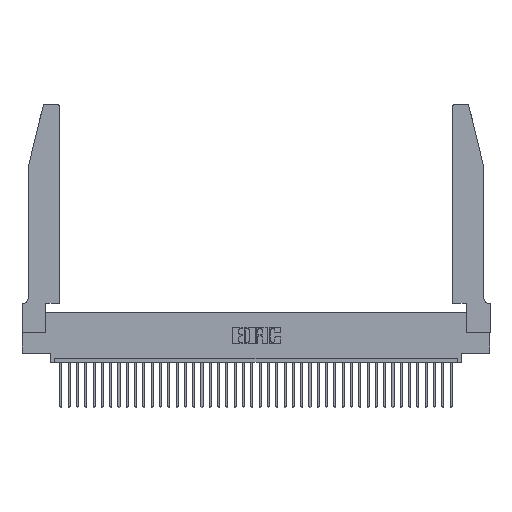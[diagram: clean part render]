
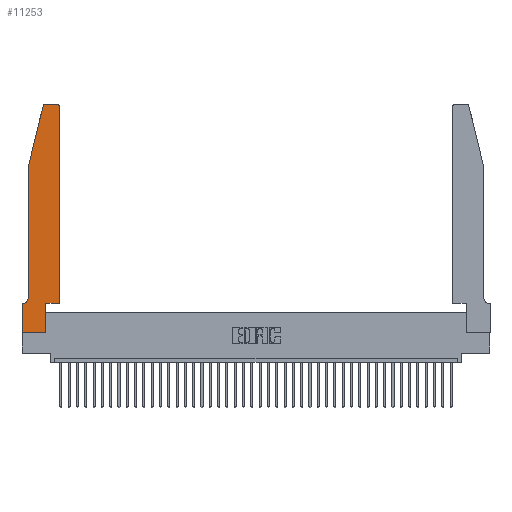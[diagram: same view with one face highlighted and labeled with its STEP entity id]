
A CAD part, top view. The second image highlights one B-rep face of the part: STEP entity #11253.
In plain terms, the highlighted planar face has unit normal (0, 0, 1).
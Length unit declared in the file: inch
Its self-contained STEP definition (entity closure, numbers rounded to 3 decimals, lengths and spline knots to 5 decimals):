
#1245 = EDGE_CURVE ( 'NONE', #4310, #39104, #9713, .T. ) ;
#1651 = CARTESIAN_POINT ( 'NONE',  ( 0.4505, 0.35, 0.37 ) ) ;
#2006 = VECTOR ( 'NONE', #34312, 39.37008 ) ;
#2778 = CARTESIAN_POINT ( 'NONE',  ( 0.2865, 0.35, 0.37 ) ) ;
#3630 = VERTEX_POINT ( 'NONE', #25578 ) ;
#3681 = CARTESIAN_POINT ( 'NONE',  ( 0.0755, 0.35, 0.37 ) ) ;
#4012 = DIRECTION ( 'NONE',  ( 0., 0., 1. ) ) ;
#4310 = VERTEX_POINT ( 'NONE', #18107 ) ;
#4346 = ORIENTED_EDGE ( 'NONE', *, *, #28639, .T. ) ;
#5297 = ORIENTED_EDGE ( 'NONE', *, *, #17449, .T. ) ;
#5808 = VECTOR ( 'NONE', #20023, 39.37008 ) ;
#6354 = ORIENTED_EDGE ( 'NONE', *, *, #28395, .T. ) ;
#6500 = VECTOR ( 'NONE', #26506, 39.37008 ) ;
#6659 = VERTEX_POINT ( 'NONE', #11043 ) ;
#6855 = CARTESIAN_POINT ( 'NONE',  ( 0.0055, 0.42, 0.37 ) ) ;
#7603 = DIRECTION ( 'NONE',  ( 1., 0., 0. ) ) ;
#8012 = CARTESIAN_POINT ( 'NONE',  ( 0.2865, 0.35, 0.37 ) ) ;
#9073 = LINE ( 'NONE', #1651, #40133 ) ;
#9585 = CARTESIAN_POINT ( 'NONE',  ( 0.4505, 2.72, 0.37 ) ) ;
#9713 = LINE ( 'NONE', #3681, #17056 ) ;
#10082 = DIRECTION ( 'NONE',  ( -1., 0., 0. ) ) ;
#10747 = CARTESIAN_POINT ( 'NONE',  ( 0.0755, 2., 0.37 ) ) ;
#11043 = CARTESIAN_POINT ( 'NONE',  ( 0.0755, 0.42, 0.37 ) ) ;
#11166 = CARTESIAN_POINT ( 'NONE',  ( 0.4205, 2.72, 0.37 ) ) ;
#11253 = ADVANCED_FACE ( 'NONE', ( #39019 ), #39192, .T. ) ;
#11574 = CARTESIAN_POINT ( 'NONE',  ( 0.25487, 2.72718, 0.37 ) ) ;
#12387 = LINE ( 'NONE', #8012, #6500 ) ;
#12405 = LINE ( 'NONE', #31126, #32309 ) ;
#12413 = DIRECTION ( 'NONE',  ( 0., -1., 0. ) ) ;
#12526 = DIRECTION ( 'NONE',  ( 0., -1., 0. ) ) ;
#12541 = ORIENTED_EDGE ( 'NONE', *, *, #20061, .T. ) ;
#12631 = CARTESIAN_POINT ( 'NONE',  ( 0., 0., 0.37 ) ) ;
#13280 = DIRECTION ( 'NONE',  ( -1., 0., 0. ) ) ;
#15090 = CIRCLE ( 'NONE', #30594, 0.03 ) ;
#15318 = AXIS2_PLACEMENT_3D ( 'NONE', #11166, #16724, #19846 ) ;
#15451 = ORIENTED_EDGE ( 'NONE', *, *, #33954, .T. ) ;
#16715 = ORIENTED_EDGE ( 'NONE', *, *, #1245, .T. ) ;
#16724 = DIRECTION ( 'NONE',  ( 0., 0., 1. ) ) ;
#17056 = VECTOR ( 'NONE', #10082, 39.37008 ) ;
#17449 = EDGE_CURVE ( 'NONE', #39104, #19648, #27063, .T. ) ;
#17570 = LINE ( 'NONE', #12631, #2006 ) ;
#18107 = CARTESIAN_POINT ( 'NONE',  ( 0.0055, 0.35, 0.37 ) ) ;
#18653 = ORIENTED_EDGE ( 'NONE', *, *, #20448, .T. ) ;
#18967 = ORIENTED_EDGE ( 'NONE', *, *, #39548, .T. ) ;
#19499 = CARTESIAN_POINT ( 'NONE',  ( 0.284, 2.72, 0.37 ) ) ;
#19648 = VERTEX_POINT ( 'NONE', #33228 ) ;
#19846 = DIRECTION ( 'NONE',  ( 1., 0., 0. ) ) ;
#20023 = DIRECTION ( 'NONE',  ( -0.239, -0.971, 0. ) ) ;
#20061 = EDGE_CURVE ( 'NONE', #19648, #30337, #17570, .T. ) ;
#20264 = CARTESIAN_POINT ( 'NONE',  ( 0., 0.35, 0.37 ) ) ;
#20448 = EDGE_CURVE ( 'NONE', #33171, #39243, #30648, .T. ) ;
#20653 = DIRECTION ( 'NONE',  ( 1., 0., 0. ) ) ;
#21458 = LINE ( 'NONE', #29177, #23873 ) ;
#21601 = CARTESIAN_POINT ( 'NONE',  ( 0.284, 2.75, 0.37 ) ) ;
#22159 = AXIS2_PLACEMENT_3D ( 'NONE', #6855, #28776, #13280 ) ;
#22890 = DIRECTION ( 'NONE',  ( 0., 1., 0. ) ) ;
#23701 = EDGE_CURVE ( 'NONE', #34258, #3630, #34339, .T. ) ;
#23873 = VECTOR ( 'NONE', #22890, 39.37008 ) ;
#25033 = EDGE_LOOP ( 'NONE', ( #18967, #4346, #18653, #26912, #28818, #16715, #5297, #12541, #28242, #15451, #6354, #25259 ) ) ;
#25255 = EDGE_CURVE ( 'NONE', #39243, #6659, #12405, .T. ) ;
#25259 = ORIENTED_EDGE ( 'NONE', *, *, #23701, .T. ) ;
#25514 = AXIS2_PLACEMENT_3D ( 'NONE', #26767, #29883, #20653 ) ;
#25578 = CARTESIAN_POINT ( 'NONE',  ( 0.4205, 2.75, 0.37 ) ) ;
#25828 = CARTESIAN_POINT ( 'NONE',  ( 0.0755, 2., 0.37 ) ) ;
#26227 = VECTOR ( 'NONE', #37434, 39.37008 ) ;
#26506 = DIRECTION ( 'NONE',  ( 0., 1., 0. ) ) ;
#26767 = CARTESIAN_POINT ( 'NONE',  ( 0., 0.35, 0.37 ) ) ;
#26912 = ORIENTED_EDGE ( 'NONE', *, *, #25255, .T. ) ;
#27063 = LINE ( 'NONE', #39986, #37613 ) ;
#28242 = ORIENTED_EDGE ( 'NONE', *, *, #30632, .T. ) ;
#28395 = EDGE_CURVE ( 'NONE', #37802, #34258, #21458, .T. ) ;
#28639 = EDGE_CURVE ( 'NONE', #33413, #33171, #15090, .T. ) ;
#28776 = DIRECTION ( 'NONE',  ( 0., 0., -1. ) ) ;
#28818 = ORIENTED_EDGE ( 'NONE', *, *, #37581, .T. ) ;
#29177 = CARTESIAN_POINT ( 'NONE',  ( 0.4505, 0.35, 0.37 ) ) ;
#29435 = DIRECTION ( 'NONE',  ( 1., 0., 0. ) ) ;
#29883 = DIRECTION ( 'NONE',  ( 0., 0., 1. ) ) ;
#29959 = CARTESIAN_POINT ( 'NONE',  ( 0.2865, 0., 0.37 ) ) ;
#30337 = VERTEX_POINT ( 'NONE', #29959 ) ;
#30594 = AXIS2_PLACEMENT_3D ( 'NONE', #19499, #4012, #29435 ) ;
#30632 = EDGE_CURVE ( 'NONE', #30337, #34790, #12387, .T. ) ;
#30648 = LINE ( 'NONE', #25828, #5808 ) ;
#31126 = CARTESIAN_POINT ( 'NONE',  ( 0.0755, 2., 0.37 ) ) ;
#32309 = VECTOR ( 'NONE', #12526, 39.37008 ) ;
#33171 = VERTEX_POINT ( 'NONE', #11574 ) ;
#33228 = CARTESIAN_POINT ( 'NONE',  ( 0., 0., 0.37 ) ) ;
#33413 = VERTEX_POINT ( 'NONE', #21601 ) ;
#33954 = EDGE_CURVE ( 'NONE', #34790, #37802, #9073, .T. ) ;
#34258 = VERTEX_POINT ( 'NONE', #9585 ) ;
#34312 = DIRECTION ( 'NONE',  ( 1., 0., 0. ) ) ;
#34339 = CIRCLE ( 'NONE', #15318, 0.03 ) ;
#34790 = VERTEX_POINT ( 'NONE', #2778 ) ;
#34884 = LINE ( 'NONE', #37489, #26227 ) ;
#35492 = CARTESIAN_POINT ( 'NONE',  ( 0.4505, 0.35, 0.37 ) ) ;
#37434 = DIRECTION ( 'NONE',  ( -1., 0., 0. ) ) ;
#37489 = CARTESIAN_POINT ( 'NONE',  ( 0.2605, 2.75, 0.37 ) ) ;
#37581 = EDGE_CURVE ( 'NONE', #6659, #4310, #39225, .T. ) ;
#37613 = VECTOR ( 'NONE', #12413, 39.37008 ) ;
#37802 = VERTEX_POINT ( 'NONE', #35492 ) ;
#39019 = FACE_OUTER_BOUND ( 'NONE', #25033, .T. ) ;
#39104 = VERTEX_POINT ( 'NONE', #20264 ) ;
#39192 = PLANE ( 'NONE',  #25514 ) ;
#39225 = CIRCLE ( 'NONE', #22159, 0.07 ) ;
#39243 = VERTEX_POINT ( 'NONE', #10747 ) ;
#39548 = EDGE_CURVE ( 'NONE', #3630, #33413, #34884, .T. ) ;
#39986 = CARTESIAN_POINT ( 'NONE',  ( 0., 0., 0.37 ) ) ;
#40133 = VECTOR ( 'NONE', #7603, 39.37008 ) ;
